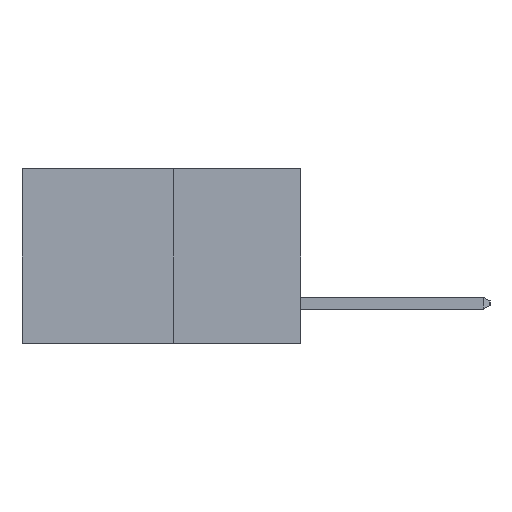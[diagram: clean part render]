
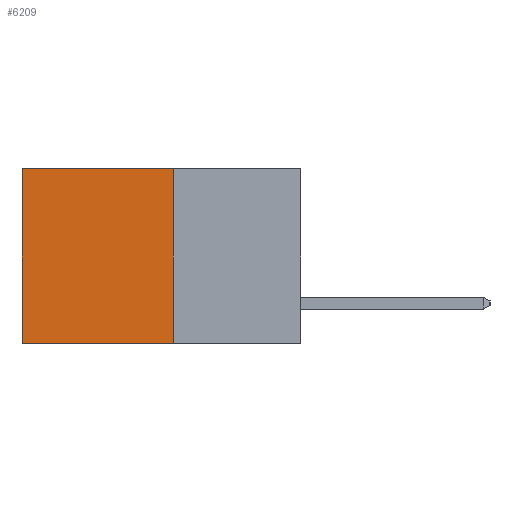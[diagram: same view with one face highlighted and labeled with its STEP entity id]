
A CAD part, left-side view. The second image highlights one B-rep face of the part: STEP entity #6209.
In plain terms, the highlighted planar face has unit normal (-1, 0, 0).
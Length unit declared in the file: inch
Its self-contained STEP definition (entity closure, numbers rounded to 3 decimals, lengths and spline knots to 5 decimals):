
#282 = ORIENTED_EDGE ( 'NONE', *, *, #4807, .F. ) ;
#645 = LINE ( 'NONE', #8444, #8931 ) ;
#1309 = VECTOR ( 'NONE', #4549, 39.37008 ) ;
#1540 = CARTESIAN_POINT ( 'NONE',  ( 0.277, 0.27, -0.37 ) ) ;
#1594 = LINE ( 'NONE', #9873, #1309 ) ;
#1966 = CARTESIAN_POINT ( 'NONE',  ( 0.277, 0.27, -0.37 ) ) ;
#1982 = DIRECTION ( 'NONE',  ( 0., 0., -1. ) ) ;
#2296 = ORIENTED_EDGE ( 'NONE', *, *, #10257, .F. ) ;
#3209 = EDGE_CURVE ( 'NONE', #8041, #4639, #645, .T. ) ;
#3252 = VERTEX_POINT ( 'NONE', #7441 ) ;
#3685 = CARTESIAN_POINT ( 'NONE',  ( 0.277, 0.59, 0. ) ) ;
#3828 = DIRECTION ( 'NONE',  ( 1., 0., 0. ) ) ;
#4189 = ORIENTED_EDGE ( 'NONE', *, *, #3209, .T. ) ;
#4198 = VECTOR ( 'NONE', #1982, 39.37008 ) ;
#4549 = DIRECTION ( 'NONE',  ( 0., 0., -1. ) ) ;
#4639 = VERTEX_POINT ( 'NONE', #3685 ) ;
#4786 = AXIS2_PLACEMENT_3D ( 'NONE', #5394, #3828, #9216 ) ;
#4807 = EDGE_CURVE ( 'NONE', #8041, #3252, #8528, .T. ) ;
#5194 = FACE_OUTER_BOUND ( 'NONE', #9324, .T. ) ;
#5394 = CARTESIAN_POINT ( 'NONE',  ( 0.277, 0.27, -0.37 ) ) ;
#5912 = VERTEX_POINT ( 'NONE', #9583 ) ;
#6159 = EDGE_CURVE ( 'NONE', #4639, #5912, #1594, .T. ) ;
#6209 = ADVANCED_FACE ( 'NONE', ( #5194 ), #6933, .F. ) ;
#6933 = PLANE ( 'NONE',  #4786 ) ;
#7441 = CARTESIAN_POINT ( 'NONE',  ( 0.277, 0.27, -0.37 ) ) ;
#7832 = DIRECTION ( 'NONE',  ( 0., 1., 0. ) ) ;
#8041 = VERTEX_POINT ( 'NONE', #8138 ) ;
#8138 = CARTESIAN_POINT ( 'NONE',  ( 0.277, 0.27, 0. ) ) ;
#8444 = CARTESIAN_POINT ( 'NONE',  ( 0.277, 0.27, 0. ) ) ;
#8528 = LINE ( 'NONE', #1966, #4198 ) ;
#8864 = ORIENTED_EDGE ( 'NONE', *, *, #6159, .T. ) ;
#8931 = VECTOR ( 'NONE', #7832, 39.37008 ) ;
#9216 = DIRECTION ( 'NONE',  ( 0., 0., -1. ) ) ;
#9324 = EDGE_LOOP ( 'NONE', ( #8864, #2296, #282, #4189 ) ) ;
#9411 = DIRECTION ( 'NONE',  ( 0., 1., 0. ) ) ;
#9533 = LINE ( 'NONE', #1540, #9771 ) ;
#9583 = CARTESIAN_POINT ( 'NONE',  ( 0.277, 0.59, -0.37 ) ) ;
#9771 = VECTOR ( 'NONE', #9411, 39.37008 ) ;
#9873 = CARTESIAN_POINT ( 'NONE',  ( 0.277, 0.59, -0.37 ) ) ;
#10257 = EDGE_CURVE ( 'NONE', #3252, #5912, #9533, .T. ) ;
